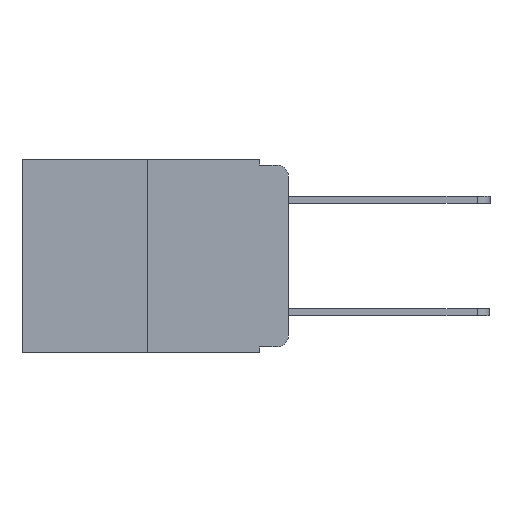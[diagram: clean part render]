
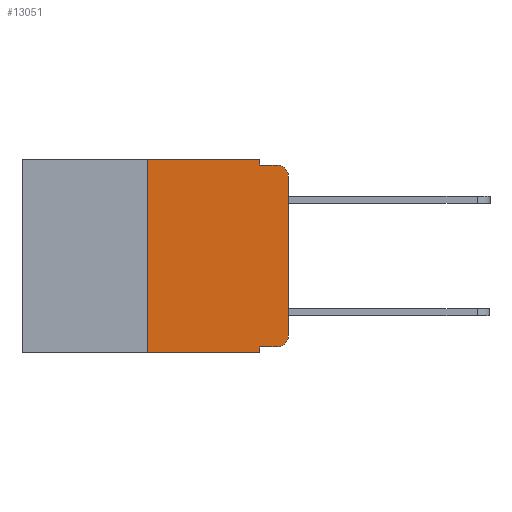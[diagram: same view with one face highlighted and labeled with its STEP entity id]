
A CAD part, left-side view. The second image highlights one B-rep face of the part: STEP entity #13051.
In plain terms, the highlighted planar face has unit normal (-1, 0, 0).
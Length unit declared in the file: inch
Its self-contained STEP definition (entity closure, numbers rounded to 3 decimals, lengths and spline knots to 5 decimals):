
#185 = LINE ( 'NONE', #17021, #8021 ) ;
#257 = EDGE_CURVE ( 'NONE', #3304, #2567, #12001, .T. ) ;
#267 = VECTOR ( 'NONE', #4936, 39.37008 ) ;
#357 = CARTESIAN_POINT ( 'NONE',  ( 0., 0.02, -0.333 ) ) ;
#566 = LINE ( 'NONE', #16093, #8345 ) ;
#773 = CARTESIAN_POINT ( 'NONE',  ( 0., 0.02, -0.313 ) ) ;
#905 = VERTEX_POINT ( 'NONE', #16617 ) ;
#1257 = ORIENTED_EDGE ( 'NONE', *, *, #10449, .F. ) ;
#1599 = ORIENTED_EDGE ( 'NONE', *, *, #2464, .F. ) ;
#2155 = VERTEX_POINT ( 'NONE', #7413 ) ;
#2167 = PLANE ( 'NONE',  #15257 ) ;
#2377 = CARTESIAN_POINT ( 'NONE',  ( 0., 0.473, 0. ) ) ;
#2417 = DIRECTION ( 'NONE',  ( 0., 0., -1. ) ) ;
#2464 = EDGE_CURVE ( 'NONE', #8974, #905, #15625, .T. ) ;
#2567 = VERTEX_POINT ( 'NONE', #6279 ) ;
#2915 = EDGE_CURVE ( 'NONE', #905, #4316, #4500, .T. ) ;
#3024 = VERTEX_POINT ( 'NONE', #14821 ) ;
#3304 = VERTEX_POINT ( 'NONE', #11553 ) ;
#3400 = CARTESIAN_POINT ( 'NONE',  ( 0., 0.051, -0.333 ) ) ;
#3762 = DIRECTION ( 'NONE',  ( 1., 0., 0. ) ) ;
#3777 = ORIENTED_EDGE ( 'NONE', *, *, #9540, .F. ) ;
#4139 = FACE_OUTER_BOUND ( 'NONE', #10068, .T. ) ;
#4316 = VERTEX_POINT ( 'NONE', #14111 ) ;
#4500 = LINE ( 'NONE', #2377, #15202 ) ;
#4936 = DIRECTION ( 'NONE',  ( 0., 0., -1. ) ) ;
#5398 = VERTEX_POINT ( 'NONE', #5938 ) ;
#5611 = EDGE_CURVE ( 'NONE', #4316, #5398, #185, .T. ) ;
#5739 = ORIENTED_EDGE ( 'NONE', *, *, #15751, .T. ) ;
#5816 = VECTOR ( 'NONE', #17025, 39.37008 ) ;
#5938 = CARTESIAN_POINT ( 'NONE',  ( 0., 0.051, -0.01 ) ) ;
#6137 = CARTESIAN_POINT ( 'NONE',  ( 0., 0.051, -0.01 ) ) ;
#6279 = CARTESIAN_POINT ( 'NONE',  ( 0., 0.02, -0.01 ) ) ;
#6956 = VECTOR ( 'NONE', #7947, 39.37008 ) ;
#7128 = CARTESIAN_POINT ( 'NONE',  ( 0., 0., 0. ) ) ;
#7413 = CARTESIAN_POINT ( 'NONE',  ( 0., 0.051, -0.333 ) ) ;
#7816 = ORIENTED_EDGE ( 'NONE', *, *, #17853, .T. ) ;
#7904 = CARTESIAN_POINT ( 'NONE',  ( 0., 0.051, 0. ) ) ;
#7947 = DIRECTION ( 'NONE',  ( 0., -1., 0. ) ) ;
#8021 = VECTOR ( 'NONE', #8058, 39.37008 ) ;
#8041 = VECTOR ( 'NONE', #8622, 39.37008 ) ;
#8058 = DIRECTION ( 'NONE',  ( 0., 0., -1. ) ) ;
#8297 = ORIENTED_EDGE ( 'NONE', *, *, #257, .T. ) ;
#8345 = VECTOR ( 'NONE', #9489, 39.37008 ) ;
#8622 = DIRECTION ( 'NONE',  ( 0., 0., 1. ) ) ;
#8974 = VERTEX_POINT ( 'NONE', #13539 ) ;
#8985 = VERTEX_POINT ( 'NONE', #357 ) ;
#9489 = DIRECTION ( 'NONE',  ( 0., -1., 0. ) ) ;
#9540 = EDGE_CURVE ( 'NONE', #5398, #2567, #16310, .T. ) ;
#9556 = DIRECTION ( 'NONE',  ( 0., 0., 1. ) ) ;
#9703 = CARTESIAN_POINT ( 'NONE',  ( 0., 0.473, 0. ) ) ;
#9751 = EDGE_CURVE ( 'NONE', #8974, #3024, #566, .T. ) ;
#9851 = ORIENTED_EDGE ( 'NONE', *, *, #14864, .T. ) ;
#10068 = EDGE_LOOP ( 'NONE', ( #7816, #8297, #3777, #10688, #12330, #1599, #10665, #1257, #9851, #5739 ) ) ;
#10449 = EDGE_CURVE ( 'NONE', #2155, #3024, #12133, .T. ) ;
#10665 = ORIENTED_EDGE ( 'NONE', *, *, #9751, .T. ) ;
#10688 = ORIENTED_EDGE ( 'NONE', *, *, #5611, .F. ) ;
#11245 = DIRECTION ( 'NONE',  ( -1., 0., 0. ) ) ;
#11532 = CIRCLE ( 'NONE', #11757, 0.02 ) ;
#11553 = CARTESIAN_POINT ( 'NONE',  ( 0., 0., -0.03 ) ) ;
#11692 = LINE ( 'NONE', #7128, #8041 ) ;
#11757 = AXIS2_PLACEMENT_3D ( 'NONE', #773, #11245, #2417 ) ;
#12001 = CIRCLE ( 'NONE', #15163, 0.02 ) ;
#12133 = LINE ( 'NONE', #7904, #267 ) ;
#12330 = ORIENTED_EDGE ( 'NONE', *, *, #2915, .F. ) ;
#13051 = ADVANCED_FACE ( 'NONE', ( #4139 ), #2167, .F. ) ;
#13370 = DIRECTION ( 'NONE',  ( -1., 0., 0. ) ) ;
#13539 = CARTESIAN_POINT ( 'NONE',  ( 0., 0.25, -0.343 ) ) ;
#13665 = DIRECTION ( 'NONE',  ( 0., 0., -1. ) ) ;
#14111 = CARTESIAN_POINT ( 'NONE',  ( 0., 0.051, 0. ) ) ;
#14630 = LINE ( 'NONE', #3400, #6956 ) ;
#14821 = CARTESIAN_POINT ( 'NONE',  ( 0., 0.051, -0.343 ) ) ;
#14864 = EDGE_CURVE ( 'NONE', #2155, #8985, #14630, .T. ) ;
#15163 = AXIS2_PLACEMENT_3D ( 'NONE', #15907, #13370, #18325 ) ;
#15191 = CARTESIAN_POINT ( 'NONE',  ( 0., 0.25, 0. ) ) ;
#15202 = VECTOR ( 'NONE', #17030, 39.37008 ) ;
#15257 = AXIS2_PLACEMENT_3D ( 'NONE', #9703, #3762, #13665 ) ;
#15625 = LINE ( 'NONE', #15191, #18321 ) ;
#15751 = EDGE_CURVE ( 'NONE', #8985, #18451, #11532, .T. ) ;
#15907 = CARTESIAN_POINT ( 'NONE',  ( 0., 0.02, -0.03 ) ) ;
#16093 = CARTESIAN_POINT ( 'NONE',  ( 0., 0.473, -0.343 ) ) ;
#16310 = LINE ( 'NONE', #6137, #5816 ) ;
#16407 = CARTESIAN_POINT ( 'NONE',  ( 0., 0., -0.313 ) ) ;
#16617 = CARTESIAN_POINT ( 'NONE',  ( 0., 0.25, 0. ) ) ;
#17021 = CARTESIAN_POINT ( 'NONE',  ( 0., 0.051, 0. ) ) ;
#17025 = DIRECTION ( 'NONE',  ( 0., -1., 0. ) ) ;
#17030 = DIRECTION ( 'NONE',  ( 0., -1., 0. ) ) ;
#17853 = EDGE_CURVE ( 'NONE', #18451, #3304, #11692, .T. ) ;
#18321 = VECTOR ( 'NONE', #9556, 39.37008 ) ;
#18325 = DIRECTION ( 'NONE',  ( 0., 0., -1. ) ) ;
#18451 = VERTEX_POINT ( 'NONE', #16407 ) ;
